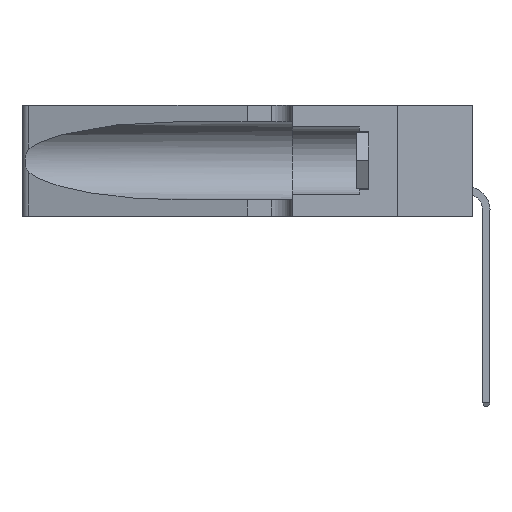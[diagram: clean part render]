
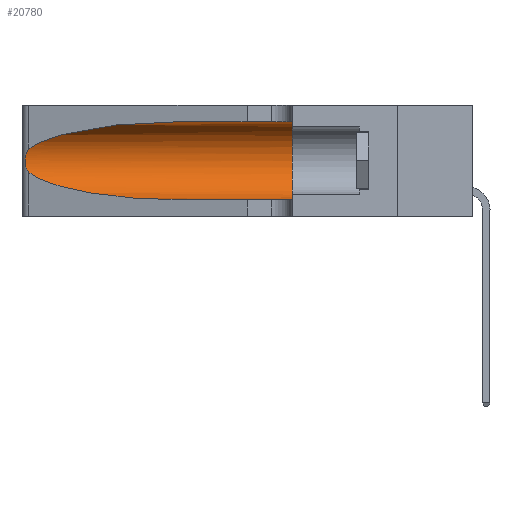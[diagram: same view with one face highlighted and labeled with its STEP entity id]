
A CAD part, left-side view. The second image highlights one B-rep face of the part: STEP entity #20780.
In plain terms, the highlighted cylindrical face has radius 3.308 mm (diameter 6.617 mm), a partial arc.
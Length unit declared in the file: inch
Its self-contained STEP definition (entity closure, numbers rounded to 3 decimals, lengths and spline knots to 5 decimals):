
#213 = DIRECTION ( 'NONE',  ( 0., 0., 1. ) ) ;
#440 = CARTESIAN_POINT ( 'NONE',  ( 0.25487, 1.22718, 0.22369 ) ) ;
#457 =( BOUNDED_CURVE ( )  B_SPLINE_CURVE ( 3, ( #20978, #17753, #13994, #8939 ),
 .UNSPECIFIED., .F., .F. ) 
 B_SPLINE_CURVE_WITH_KNOTS ( ( 4, 4 ),
 ( 3.44316, 4.71239 ),
 .UNSPECIFIED. ) 
 CURVE ( )  GEOMETRIC_REPRESENTATION_ITEM ( )  RATIONAL_B_SPLINE_CURVE ( ( 1., 0.87, 0.87, 1. ) ) 
 REPRESENTATION_ITEM ( '' )  );
#497 = CARTESIAN_POINT ( 'NONE',  ( 0.25787, 1.23484, 0.2124 ) ) ;
#513 = ORIENTED_EDGE ( 'NONE', *, *, #6867, .T. ) ;
#1217 = CARTESIAN_POINT ( 'NONE',  ( 0.1305, 1.61858, 0.05475 ) ) ;
#1416 = CARTESIAN_POINT ( 'NONE',  ( 0.1305, 0.35, 0.31525 ) ) ;
#1672 = CARTESIAN_POINT ( 'NONE',  ( 0.25487, 1.22718, 0.14631 ) ) ;
#2120 = DIRECTION ( 'NONE',  ( 0., -1., 0. ) ) ;
#2186 = CARTESIAN_POINT ( 'NONE',  ( 0.25555, 1.22994, 0.2215 ) ) ;
#2432 = LINE ( 'NONE', #13964, #4333 ) ;
#3223 = CARTESIAN_POINT ( 'NONE',  ( 0.25856, 1.23593, 0.16098 ) ) ;
#3278 = CARTESIAN_POINT ( 'NONE',  ( 0.1305, 0.72297, 0.31525 ) ) ;
#3371 = CARTESIAN_POINT ( 'NONE',  ( 0.25789, 1.23486, 0.15765 ) ) ;
#3935 = CARTESIAN_POINT ( 'NONE',  ( 0.25639, 1.23184, 0.21858 ) ) ;
#4312 = CYLINDRICAL_SURFACE ( 'NONE', #12413, 0.13025 ) ;
#4333 = VECTOR ( 'NONE', #2120, 39.37008 ) ;
#5098 = CARTESIAN_POINT ( 'NONE',  ( 0.26017, 1.23833, 0.17102 ) ) ;
#5295 = CARTESIAN_POINT ( 'NONE',  ( 0.18966, 0.96281, 0.31525 ) ) ;
#5638 = ORIENTED_EDGE ( 'NONE', *, *, #19958, .T. ) ;
#6427 = VERTEX_POINT ( 'NONE', #21422 ) ;
#6578 = AXIS2_PLACEMENT_3D ( 'NONE', #8806, #17334, #213 ) ;
#6601 = VERTEX_POINT ( 'NONE', #19952 ) ;
#6682 = VERTEX_POINT ( 'NONE', #19790 ) ;
#6772 = ORIENTED_EDGE ( 'NONE', *, *, #19190, .T. ) ;
#6867 = EDGE_CURVE ( 'NONE', #6682, #6601, #12824, .T. ) ;
#6894 = CARTESIAN_POINT ( 'NONE',  ( 0.26075, 1.23896, 0.19203 ) ) ;
#7528 = ORIENTED_EDGE ( 'NONE', *, *, #10732, .T. ) ;
#8806 = CARTESIAN_POINT ( 'NONE',  ( 0.1305, 0.35, 0.185 ) ) ;
#8939 = CARTESIAN_POINT ( 'NONE',  ( 0.1305, 0.72297, 0.05475 ) ) ;
#9297 = EDGE_LOOP ( 'NONE', ( #513, #7528, #5638, #6772, #19937, #15790 ) ) ;
#9843 = CARTESIAN_POINT ( 'NONE',  ( 0.1305, 1.61858, 0.185 ) ) ;
#10300 = EDGE_CURVE ( 'NONE', #6682, #12468, #2432, .T. ) ;
#10343 = CARTESIAN_POINT ( 'NONE',  ( 0.26075, 1.23896, 0.178 ) ) ;
#10732 = EDGE_CURVE ( 'NONE', #6601, #6427, #11186, .T. ) ;
#11048 = LINE ( 'NONE', #1217, #12127 ) ;
#11186 = B_SPLINE_CURVE_WITH_KNOTS ( 'NONE', 3,
 ( #440, #2186, #3935, #497, #14152, #11846, #6894, #10343, #5098, #3223, #3371, #15343, #17138, #1672 ),
 .UNSPECIFIED., .F., .F.,
 ( 4, 2, 2, 2, 2, 2, 4 ),
 ( 0., 0.00027, 0.00053, 0.00107, 0.0016, 0.00187, 0.00214 ),
 .UNSPECIFIED. ) ;
#11782 = CIRCLE ( 'NONE', #6578, 0.13025 ) ;
#11819 = FACE_OUTER_BOUND ( 'NONE', #9297, .T. ) ;
#11846 = CARTESIAN_POINT ( 'NONE',  ( 0.26018, 1.23835, 0.19895 ) ) ;
#11971 = CARTESIAN_POINT ( 'NONE',  ( 0.2373, 1.15595, 0.28018 ) ) ;
#12127 = VECTOR ( 'NONE', #21550, 39.37008 ) ;
#12413 = AXIS2_PLACEMENT_3D ( 'NONE', #9843, #15123, #16696 ) ;
#12468 = VERTEX_POINT ( 'NONE', #1416 ) ;
#12824 =( BOUNDED_CURVE ( )  B_SPLINE_CURVE ( 3, ( #3278, #5295, #11971, #15258 ),
 .UNSPECIFIED., .F., .T. ) 
 B_SPLINE_CURVE_WITH_KNOTS ( ( 4, 4 ),
 ( 1.5708, 2.84003 ),
 .UNSPECIFIED. ) 
 CURVE ( )  GEOMETRIC_REPRESENTATION_ITEM ( )  RATIONAL_B_SPLINE_CURVE ( ( 1., 0.87, 0.87, 1. ) ) 
 REPRESENTATION_ITEM ( '' )  );
#13951 = CARTESIAN_POINT ( 'NONE',  ( 0.1305, 0.35, 0.05475 ) ) ;
#13964 = CARTESIAN_POINT ( 'NONE',  ( 0.1305, 1.61858, 0.31525 ) ) ;
#13994 = CARTESIAN_POINT ( 'NONE',  ( 0.18966, 0.96281, 0.05475 ) ) ;
#14112 = VERTEX_POINT ( 'NONE', #19956 ) ;
#14152 = CARTESIAN_POINT ( 'NONE',  ( 0.25854, 1.2359, 0.20912 ) ) ;
#15123 = DIRECTION ( 'NONE',  ( 0., -1., 0. ) ) ;
#15258 = CARTESIAN_POINT ( 'NONE',  ( 0.25487, 1.22718, 0.22369 ) ) ;
#15343 = CARTESIAN_POINT ( 'NONE',  ( 0.25639, 1.23186, 0.15144 ) ) ;
#15790 = ORIENTED_EDGE ( 'NONE', *, *, #10300, .F. ) ;
#16696 = DIRECTION ( 'NONE',  ( 0., 0., -1. ) ) ;
#17138 = CARTESIAN_POINT ( 'NONE',  ( 0.25555, 1.22993, 0.14849 ) ) ;
#17334 = DIRECTION ( 'NONE',  ( 0., 1., 0. ) ) ;
#17753 = CARTESIAN_POINT ( 'NONE',  ( 0.2373, 1.15595, 0.08982 ) ) ;
#19190 = EDGE_CURVE ( 'NONE', #14112, #20983, #11048, .T. ) ;
#19790 = CARTESIAN_POINT ( 'NONE',  ( 0.1305, 0.72297, 0.31525 ) ) ;
#19937 = ORIENTED_EDGE ( 'NONE', *, *, #21796, .F. ) ;
#19952 = CARTESIAN_POINT ( 'NONE',  ( 0.25487, 1.22718, 0.22369 ) ) ;
#19956 = CARTESIAN_POINT ( 'NONE',  ( 0.1305, 0.72297, 0.05475 ) ) ;
#19958 = EDGE_CURVE ( 'NONE', #6427, #14112, #457, .T. ) ;
#20780 = ADVANCED_FACE ( 'NONE', ( #11819 ), #4312, .F. ) ;
#20978 = CARTESIAN_POINT ( 'NONE',  ( 0.25487, 1.22718, 0.14631 ) ) ;
#20983 = VERTEX_POINT ( 'NONE', #13951 ) ;
#21422 = CARTESIAN_POINT ( 'NONE',  ( 0.25487, 1.22718, 0.14631 ) ) ;
#21550 = DIRECTION ( 'NONE',  ( 0., -1., 0. ) ) ;
#21796 = EDGE_CURVE ( 'NONE', #12468, #20983, #11782, .T. ) ;
